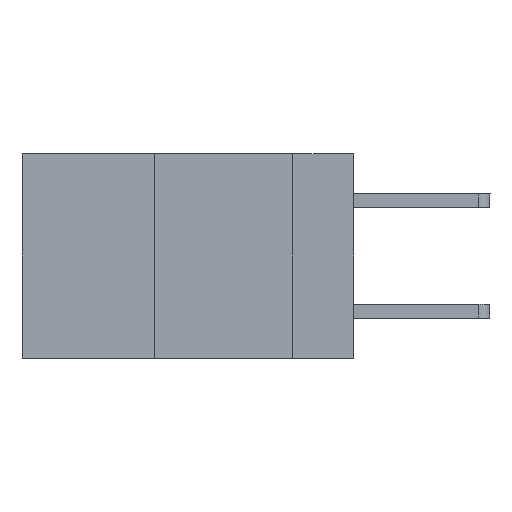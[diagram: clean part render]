
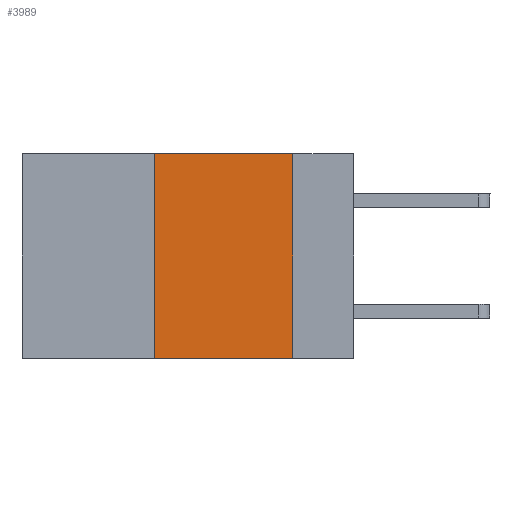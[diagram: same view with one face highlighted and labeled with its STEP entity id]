
A CAD part, left-side view. The second image highlights one B-rep face of the part: STEP entity #3989.
In plain terms, the highlighted planar face has unit normal (-1, 0, 0).
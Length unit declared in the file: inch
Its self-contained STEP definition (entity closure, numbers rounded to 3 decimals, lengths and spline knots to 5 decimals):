
#635 = LINE ( 'NONE', #8586, #5864 ) ;
#1106 = CARTESIAN_POINT ( 'NONE',  ( 0., 0.36, 0. ) ) ;
#1295 = VERTEX_POINT ( 'NONE', #10763 ) ;
#1326 = DIRECTION ( 'NONE',  ( 0., 0., -1. ) ) ;
#1567 = CARTESIAN_POINT ( 'NONE',  ( 0., 0.11, 0. ) ) ;
#1744 = EDGE_LOOP ( 'NONE', ( #7256, #7558, #7595, #7640 ) ) ;
#2325 = VERTEX_POINT ( 'NONE', #1567 ) ;
#2453 = LINE ( 'NONE', #9925, #4867 ) ;
#2693 = AXIS2_PLACEMENT_3D ( 'NONE', #11375, #13422, #7229 ) ;
#2929 = VECTOR ( 'NONE', #4570, 39.37008 ) ;
#3989 = ADVANCED_FACE ( 'NONE', ( #6194 ), #10326, .F. ) ;
#4570 = DIRECTION ( 'NONE',  ( 0., -1., 0. ) ) ;
#4799 = DIRECTION ( 'NONE',  ( 0., -1., 0. ) ) ;
#4867 = VECTOR ( 'NONE', #4799, 39.37008 ) ;
#5416 = EDGE_CURVE ( 'NONE', #7985, #1295, #2453, .T. ) ;
#5864 = VECTOR ( 'NONE', #1326, 39.37008 ) ;
#6194 = FACE_OUTER_BOUND ( 'NONE', #1744, .T. ) ;
#6539 = EDGE_CURVE ( 'NONE', #2325, #1295, #635, .T. ) ;
#7229 = DIRECTION ( 'NONE',  ( 0., 0., -1. ) ) ;
#7244 = EDGE_CURVE ( 'NONE', #10009, #2325, #8405, .T. ) ;
#7256 = ORIENTED_EDGE ( 'NONE', *, *, #6539, .F. ) ;
#7558 = ORIENTED_EDGE ( 'NONE', *, *, #7244, .F. ) ;
#7595 = ORIENTED_EDGE ( 'NONE', *, *, #10953, .F. ) ;
#7640 = ORIENTED_EDGE ( 'NONE', *, *, #5416, .T. ) ;
#7985 = VERTEX_POINT ( 'NONE', #9108 ) ;
#8405 = LINE ( 'NONE', #8656, #2929 ) ;
#8586 = CARTESIAN_POINT ( 'NONE',  ( 0., 0.11, 0. ) ) ;
#8656 = CARTESIAN_POINT ( 'NONE',  ( 0., 0.6, 0. ) ) ;
#9108 = CARTESIAN_POINT ( 'NONE',  ( 0., 0.36, -0.37 ) ) ;
#9925 = CARTESIAN_POINT ( 'NONE',  ( 0., 0.6, -0.37 ) ) ;
#10009 = VERTEX_POINT ( 'NONE', #1106 ) ;
#10326 = PLANE ( 'NONE',  #2693 ) ;
#10763 = CARTESIAN_POINT ( 'NONE',  ( 0., 0.11, -0.37 ) ) ;
#10953 = EDGE_CURVE ( 'NONE', #7985, #10009, #12675, .T. ) ;
#11375 = CARTESIAN_POINT ( 'NONE',  ( 0., 0.6, 0. ) ) ;
#11509 = DIRECTION ( 'NONE',  ( 0., 0., 1. ) ) ;
#12053 = VECTOR ( 'NONE', #11509, 39.37008 ) ;
#12540 = CARTESIAN_POINT ( 'NONE',  ( 0., 0.36, 0. ) ) ;
#12675 = LINE ( 'NONE', #12540, #12053 ) ;
#13422 = DIRECTION ( 'NONE',  ( 1., 0., 0. ) ) ;
